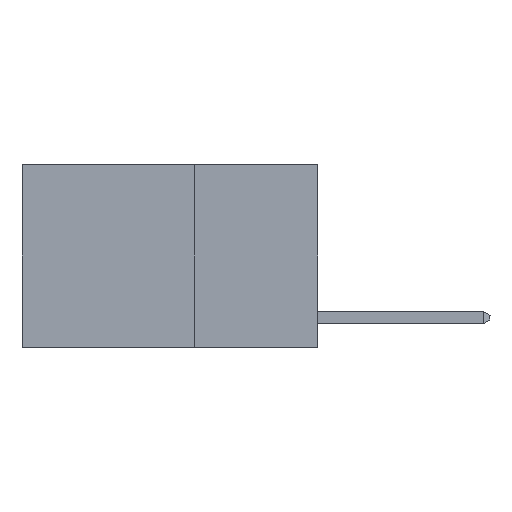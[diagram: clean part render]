
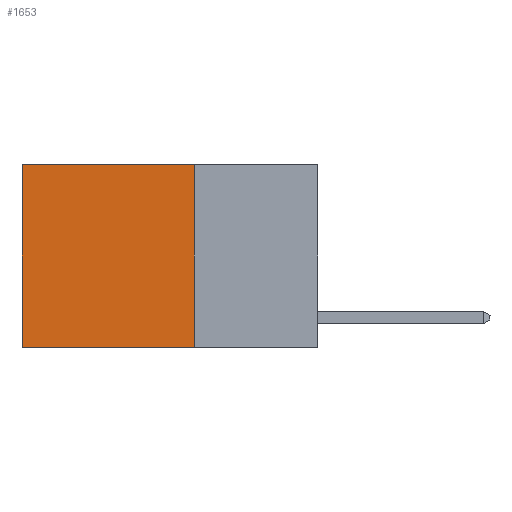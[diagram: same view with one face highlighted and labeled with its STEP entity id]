
A CAD part, left-side view. The second image highlights one B-rep face of the part: STEP entity #1653.
In plain terms, the highlighted planar face has unit normal (-1, 0, 0).
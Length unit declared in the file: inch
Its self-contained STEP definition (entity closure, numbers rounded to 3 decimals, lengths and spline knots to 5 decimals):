
#1250 = CARTESIAN_POINT ( 'NONE',  ( 0.2625, 0.25, -0.37 ) ) ;
#1271 = LINE ( 'NONE', #3886, #13001 ) ;
#1651 = PLANE ( 'NONE',  #2980 ) ;
#1653 = ADVANCED_FACE ( 'NONE', ( #3132 ), #1651, .F. ) ;
#1707 = EDGE_CURVE ( 'NONE', #3335, #7620, #8144, .T. ) ;
#1745 = CARTESIAN_POINT ( 'NONE',  ( 0.2625, 0.25, 0. ) ) ;
#1959 = LINE ( 'NONE', #1745, #12872 ) ;
#2095 = EDGE_CURVE ( 'NONE', #3335, #2897, #1959, .T. ) ;
#2215 = VERTEX_POINT ( 'NONE', #10485 ) ;
#2897 = VERTEX_POINT ( 'NONE', #10904 ) ;
#2939 = EDGE_CURVE ( 'NONE', #2897, #2215, #1271, .T. ) ;
#2980 = AXIS2_PLACEMENT_3D ( 'NONE', #11162, #12230, #7005 ) ;
#3132 = FACE_OUTER_BOUND ( 'NONE', #11747, .T. ) ;
#3297 = EDGE_CURVE ( 'NONE', #7620, #2215, #5907, .T. ) ;
#3335 = VERTEX_POINT ( 'NONE', #7524 ) ;
#3691 = CARTESIAN_POINT ( 'NONE',  ( 0.2625, 0.25, 0. ) ) ;
#3886 = CARTESIAN_POINT ( 'NONE',  ( 0.2625, 0.6, 0. ) ) ;
#4475 = VECTOR ( 'NONE', #6952, 39.37008 ) ;
#5097 = VECTOR ( 'NONE', #7758, 39.37008 ) ;
#5551 = CARTESIAN_POINT ( 'NONE',  ( 0.2625, 0.25, -0.37 ) ) ;
#5907 = LINE ( 'NONE', #1250, #5097 ) ;
#6952 = DIRECTION ( 'NONE',  ( 0., 0., -1. ) ) ;
#7005 = DIRECTION ( 'NONE',  ( 0., 0., -1. ) ) ;
#7524 = CARTESIAN_POINT ( 'NONE',  ( 0.2625, 0.25, 0. ) ) ;
#7620 = VERTEX_POINT ( 'NONE', #5551 ) ;
#7758 = DIRECTION ( 'NONE',  ( 0., 1., 0. ) ) ;
#8144 = LINE ( 'NONE', #3691, #4475 ) ;
#8182 = DIRECTION ( 'NONE',  ( 0., 1., 0. ) ) ;
#10485 = CARTESIAN_POINT ( 'NONE',  ( 0.2625, 0.6, -0.37 ) ) ;
#10552 = ORIENTED_EDGE ( 'NONE', *, *, #2939, .T. ) ;
#10904 = CARTESIAN_POINT ( 'NONE',  ( 0.2625, 0.6, 0. ) ) ;
#11162 = CARTESIAN_POINT ( 'NONE',  ( 0.2625, 0.25, 0. ) ) ;
#11747 = EDGE_LOOP ( 'NONE', ( #10552, #13047, #13677, #13402 ) ) ;
#12230 = DIRECTION ( 'NONE',  ( 1., 0., 0. ) ) ;
#12461 = DIRECTION ( 'NONE',  ( 0., 0., -1. ) ) ;
#12872 = VECTOR ( 'NONE', #8182, 39.37008 ) ;
#13001 = VECTOR ( 'NONE', #12461, 39.37008 ) ;
#13047 = ORIENTED_EDGE ( 'NONE', *, *, #3297, .F. ) ;
#13402 = ORIENTED_EDGE ( 'NONE', *, *, #2095, .T. ) ;
#13677 = ORIENTED_EDGE ( 'NONE', *, *, #1707, .F. ) ;
